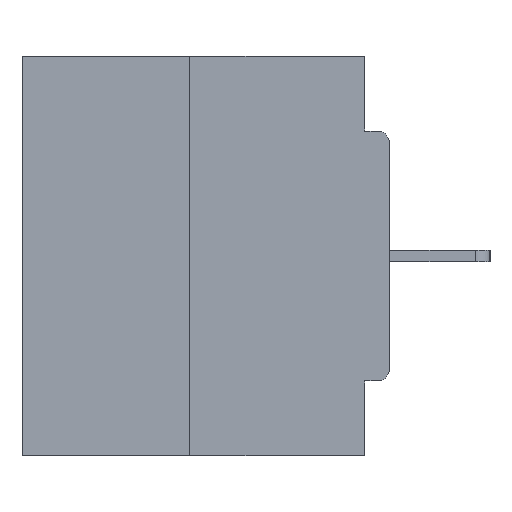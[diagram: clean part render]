
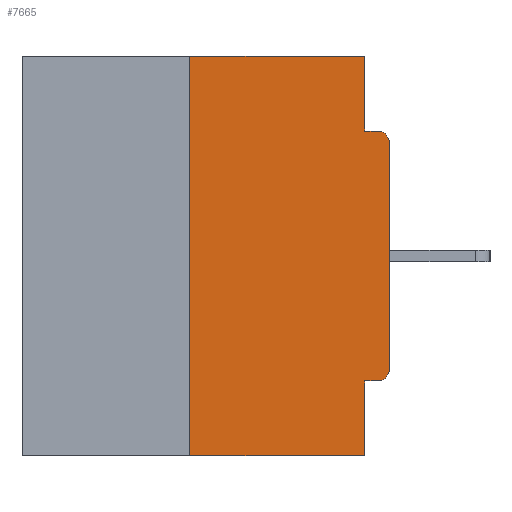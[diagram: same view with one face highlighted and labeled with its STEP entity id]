
A CAD part, left-side view. The second image highlights one B-rep face of the part: STEP entity #7665.
In plain terms, the highlighted planar face has unit normal (-1, 0, 0).
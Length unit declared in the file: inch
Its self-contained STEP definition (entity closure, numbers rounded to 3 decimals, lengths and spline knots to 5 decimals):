
#568 = CIRCLE ( 'NONE', #23762, 0.015 ) ;
#1022 = DIRECTION ( 'NONE',  ( 0., 0., 1. ) ) ;
#2995 = CARTESIAN_POINT ( 'NONE',  ( 0., 0., -0.1085 ) ) ;
#3173 = CARTESIAN_POINT ( 'NONE',  ( 0., 0., 0. ) ) ;
#3534 = CARTESIAN_POINT ( 'NONE',  ( 0., 0.015, -0.4065 ) ) ;
#3678 = VERTEX_POINT ( 'NONE', #2995 ) ;
#4023 = CARTESIAN_POINT ( 'NONE',  ( 0., 0.46, 0. ) ) ;
#4420 = DIRECTION ( 'NONE',  ( 0., 0., 1. ) ) ;
#4851 = CARTESIAN_POINT ( 'NONE',  ( 0., 0.031, 0. ) ) ;
#4952 = VECTOR ( 'NONE', #11705, 39.37008 ) ;
#5401 = VERTEX_POINT ( 'NONE', #13899 ) ;
#5547 = ORIENTED_EDGE ( 'NONE', *, *, #23080, .F. ) ;
#5867 = CARTESIAN_POINT ( 'NONE',  ( 0., 0.031, 0. ) ) ;
#6181 = ORIENTED_EDGE ( 'NONE', *, *, #20798, .F. ) ;
#6456 = DIRECTION ( 'NONE',  ( -1., 0., 0. ) ) ;
#6779 = EDGE_CURVE ( 'NONE', #5401, #19319, #10066, .T. ) ;
#6975 = DIRECTION ( 'NONE',  ( 0., 0., -1. ) ) ;
#7110 = ORIENTED_EDGE ( 'NONE', *, *, #11876, .T. ) ;
#7365 = EDGE_LOOP ( 'NONE', ( #10610, #26659, #29246, #5547, #13546, #22623, #7110, #20482, #28183, #6181 ) ) ;
#7665 = ADVANCED_FACE ( 'NONE', ( #12215 ), #10402, .F. ) ;
#7784 = CARTESIAN_POINT ( 'NONE',  ( 0., 0., -0.0935 ) ) ;
#8492 = CARTESIAN_POINT ( 'NONE',  ( 0., 0.46, -0.5 ) ) ;
#9043 = EDGE_CURVE ( 'NONE', #26681, #24987, #15400, .T. ) ;
#9082 = EDGE_CURVE ( 'NONE', #20095, #24994, #29162, .T. ) ;
#9430 = DIRECTION ( 'NONE',  ( 0., 0., -1. ) ) ;
#9555 = VECTOR ( 'NONE', #1022, 39.37008 ) ;
#9845 = LINE ( 'NONE', #4851, #13159 ) ;
#10066 = LINE ( 'NONE', #7784, #20475 ) ;
#10402 = PLANE ( 'NONE',  #17130 ) ;
#10610 = ORIENTED_EDGE ( 'NONE', *, *, #9043, .F. ) ;
#10652 = CARTESIAN_POINT ( 'NONE',  ( 0., 0.031, -0.5 ) ) ;
#11065 = LINE ( 'NONE', #8492, #22697 ) ;
#11561 = LINE ( 'NONE', #23187, #4952 ) ;
#11670 = DIRECTION ( 'NONE',  ( 0., 0., -1. ) ) ;
#11705 = DIRECTION ( 'NONE',  ( 0., 1., 0. ) ) ;
#11876 = EDGE_CURVE ( 'NONE', #24994, #3678, #23897, .T. ) ;
#12036 = DIRECTION ( 'NONE',  ( 0., -1., 0. ) ) ;
#12215 = FACE_OUTER_BOUND ( 'NONE', #7365, .T. ) ;
#13159 = VECTOR ( 'NONE', #11670, 39.37008 ) ;
#13546 = ORIENTED_EDGE ( 'NONE', *, *, #22669, .F. ) ;
#13845 = EDGE_CURVE ( 'NONE', #26325, #26681, #18201, .T. ) ;
#13899 = CARTESIAN_POINT ( 'NONE',  ( 0., 0.031, -0.0935 ) ) ;
#14359 = EDGE_CURVE ( 'NONE', #26325, #29173, #11065, .T. ) ;
#15400 = LINE ( 'NONE', #4023, #19545 ) ;
#15435 = VECTOR ( 'NONE', #4420, 39.37008 ) ;
#15687 = DIRECTION ( 'NONE',  ( 0., 0., -1. ) ) ;
#16056 = LINE ( 'NONE', #18333, #23786 ) ;
#16171 = AXIS2_PLACEMENT_3D ( 'NONE', #22782, #6456, #15687 ) ;
#16974 = CARTESIAN_POINT ( 'NONE',  ( 0., 0.015, -0.0935 ) ) ;
#17130 = AXIS2_PLACEMENT_3D ( 'NONE', #17355, #26125, #21449 ) ;
#17355 = CARTESIAN_POINT ( 'NONE',  ( 0., 0.46, 0. ) ) ;
#17504 = CARTESIAN_POINT ( 'NONE',  ( 0., 0., -0.3915 ) ) ;
#18201 = LINE ( 'NONE', #21886, #15435 ) ;
#18333 = CARTESIAN_POINT ( 'NONE',  ( 0., 0.031, -0.5 ) ) ;
#19319 = VERTEX_POINT ( 'NONE', #16974 ) ;
#19545 = VECTOR ( 'NONE', #24458, 39.37008 ) ;
#20095 = VERTEX_POINT ( 'NONE', #3534 ) ;
#20475 = VECTOR ( 'NONE', #12036, 39.37008 ) ;
#20482 = ORIENTED_EDGE ( 'NONE', *, *, #22649, .T. ) ;
#20798 = EDGE_CURVE ( 'NONE', #24987, #5401, #9845, .T. ) ;
#21449 = DIRECTION ( 'NONE',  ( 0., 0., -1. ) ) ;
#21658 = CARTESIAN_POINT ( 'NONE',  ( 0., 0.25, -0.5 ) ) ;
#21886 = CARTESIAN_POINT ( 'NONE',  ( 0., 0.25, 0. ) ) ;
#22556 = VERTEX_POINT ( 'NONE', #29830 ) ;
#22623 = ORIENTED_EDGE ( 'NONE', *, *, #9082, .T. ) ;
#22649 = EDGE_CURVE ( 'NONE', #3678, #19319, #568, .T. ) ;
#22669 = EDGE_CURVE ( 'NONE', #20095, #22556, #11561, .T. ) ;
#22697 = VECTOR ( 'NONE', #29471, 39.37008 ) ;
#22744 = DIRECTION ( 'NONE',  ( -1., 0., 0. ) ) ;
#22782 = CARTESIAN_POINT ( 'NONE',  ( 0., 0.015, -0.3915 ) ) ;
#23080 = EDGE_CURVE ( 'NONE', #22556, #29173, #16056, .T. ) ;
#23187 = CARTESIAN_POINT ( 'NONE',  ( 0., 0., -0.4065 ) ) ;
#23762 = AXIS2_PLACEMENT_3D ( 'NONE', #25017, #22744, #9430 ) ;
#23786 = VECTOR ( 'NONE', #6975, 39.37008 ) ;
#23897 = LINE ( 'NONE', #3173, #9555 ) ;
#24458 = DIRECTION ( 'NONE',  ( 0., -1., 0. ) ) ;
#24987 = VERTEX_POINT ( 'NONE', #5867 ) ;
#24994 = VERTEX_POINT ( 'NONE', #17504 ) ;
#25017 = CARTESIAN_POINT ( 'NONE',  ( 0., 0.015, -0.1085 ) ) ;
#26125 = DIRECTION ( 'NONE',  ( 1., 0., 0. ) ) ;
#26325 = VERTEX_POINT ( 'NONE', #21658 ) ;
#26659 = ORIENTED_EDGE ( 'NONE', *, *, #13845, .F. ) ;
#26681 = VERTEX_POINT ( 'NONE', #27200 ) ;
#27200 = CARTESIAN_POINT ( 'NONE',  ( 0., 0.25, 0. ) ) ;
#28183 = ORIENTED_EDGE ( 'NONE', *, *, #6779, .F. ) ;
#29162 = CIRCLE ( 'NONE', #16171, 0.015 ) ;
#29173 = VERTEX_POINT ( 'NONE', #10652 ) ;
#29246 = ORIENTED_EDGE ( 'NONE', *, *, #14359, .T. ) ;
#29471 = DIRECTION ( 'NONE',  ( 0., -1., 0. ) ) ;
#29830 = CARTESIAN_POINT ( 'NONE',  ( 0., 0.031, -0.4065 ) ) ;
